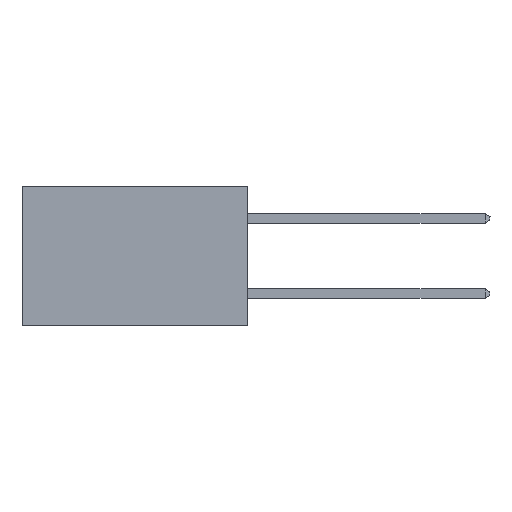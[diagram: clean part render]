
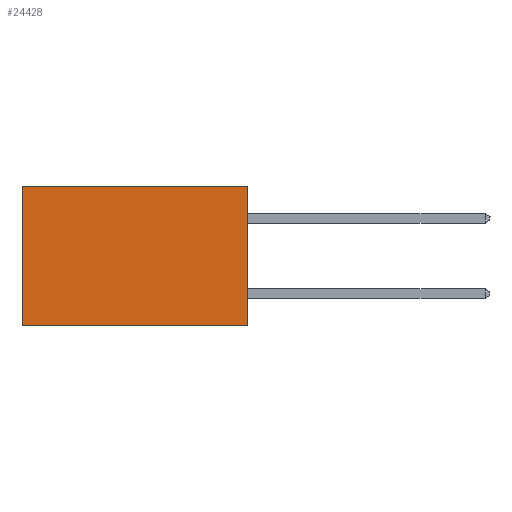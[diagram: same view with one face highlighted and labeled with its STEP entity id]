
A CAD part, left-side view. The second image highlights one B-rep face of the part: STEP entity #24428.
In plain terms, the highlighted planar face has unit normal (-1, 0, 0).
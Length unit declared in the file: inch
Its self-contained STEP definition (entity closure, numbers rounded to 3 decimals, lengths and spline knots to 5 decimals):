
#796 = LINE ( 'NONE', #3723, #25589 ) ;
#1375 = LINE ( 'NONE', #13629, #19916 ) ;
#1804 = VECTOR ( 'NONE', #3115, 39.37008 ) ;
#2640 = EDGE_CURVE ( 'NONE', #8153, #16516, #3801, .T. ) ;
#3115 = DIRECTION ( 'NONE',  ( 0., 1., 0. ) ) ;
#3723 = CARTESIAN_POINT ( 'NONE',  ( 0.298, 0., 0. ) ) ;
#3801 = LINE ( 'NONE', #18581, #28434 ) ;
#3821 = CARTESIAN_POINT ( 'NONE',  ( 0.298, 0., 0. ) ) ;
#4523 = DIRECTION ( 'NONE',  ( 0., 1., 0. ) ) ;
#6729 = VERTEX_POINT ( 'NONE', #13684 ) ;
#6990 = EDGE_CURVE ( 'NONE', #7484, #8153, #796, .T. ) ;
#7484 = VERTEX_POINT ( 'NONE', #20649 ) ;
#8153 = VERTEX_POINT ( 'NONE', #12529 ) ;
#9284 = CARTESIAN_POINT ( 'NONE',  ( 0.298, 0.6, -0.37 ) ) ;
#9370 = EDGE_CURVE ( 'NONE', #6729, #16516, #14762, .T. ) ;
#9597 = EDGE_CURVE ( 'NONE', #7484, #6729, #1375, .T. ) ;
#9661 = ORIENTED_EDGE ( 'NONE', *, *, #9370, .F. ) ;
#11125 = DIRECTION ( 'NONE',  ( 1., 0., 0. ) ) ;
#12529 = CARTESIAN_POINT ( 'NONE',  ( 0.298, 0.6, 0. ) ) ;
#13629 = CARTESIAN_POINT ( 'NONE',  ( 0.298, 0., 0. ) ) ;
#13684 = CARTESIAN_POINT ( 'NONE',  ( 0.298, 0., -0.37 ) ) ;
#13744 = ORIENTED_EDGE ( 'NONE', *, *, #6990, .T. ) ;
#14335 = ORIENTED_EDGE ( 'NONE', *, *, #9597, .F. ) ;
#14762 = LINE ( 'NONE', #15210, #1804 ) ;
#15210 = CARTESIAN_POINT ( 'NONE',  ( 0.298, 0., -0.37 ) ) ;
#16516 = VERTEX_POINT ( 'NONE', #9284 ) ;
#17110 = AXIS2_PLACEMENT_3D ( 'NONE', #3821, #11125, #27705 ) ;
#18253 = FACE_OUTER_BOUND ( 'NONE', #18314, .T. ) ;
#18314 = EDGE_LOOP ( 'NONE', ( #20584, #9661, #14335, #13744 ) ) ;
#18581 = CARTESIAN_POINT ( 'NONE',  ( 0.298, 0.6, 0. ) ) ;
#18799 = DIRECTION ( 'NONE',  ( 0., 0., -1. ) ) ;
#19916 = VECTOR ( 'NONE', #20772, 39.37008 ) ;
#20584 = ORIENTED_EDGE ( 'NONE', *, *, #2640, .T. ) ;
#20649 = CARTESIAN_POINT ( 'NONE',  ( 0.298, 0., 0. ) ) ;
#20772 = DIRECTION ( 'NONE',  ( 0., 0., -1. ) ) ;
#24428 = ADVANCED_FACE ( 'NONE', ( #18253 ), #25123, .F. ) ;
#25123 = PLANE ( 'NONE',  #17110 ) ;
#25589 = VECTOR ( 'NONE', #4523, 39.37008 ) ;
#27705 = DIRECTION ( 'NONE',  ( 0., 0., -1. ) ) ;
#28434 = VECTOR ( 'NONE', #18799, 39.37008 ) ;
